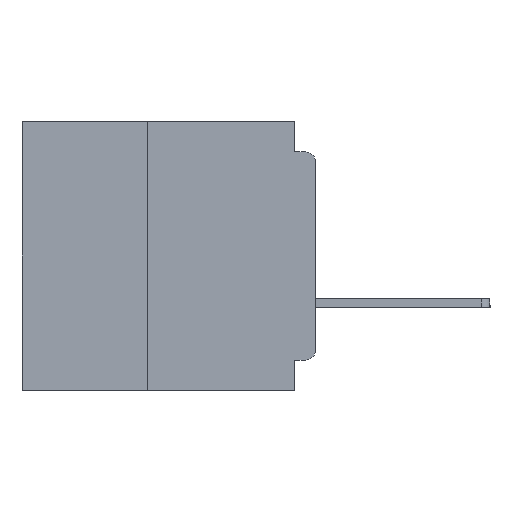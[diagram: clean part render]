
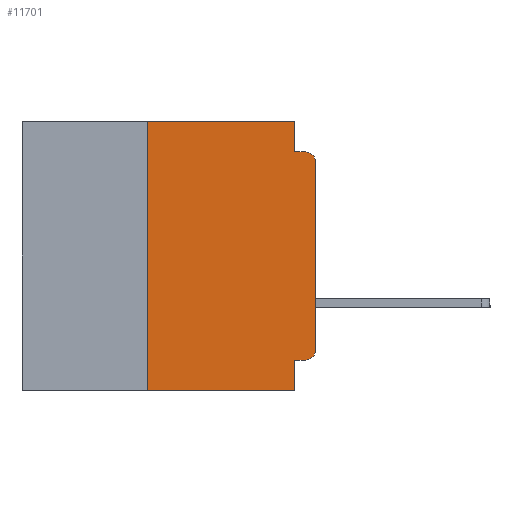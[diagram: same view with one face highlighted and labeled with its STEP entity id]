
A CAD part, left-side view. The second image highlights one B-rep face of the part: STEP entity #11701.
In plain terms, the highlighted planar face has unit normal (-1, 0, 0).
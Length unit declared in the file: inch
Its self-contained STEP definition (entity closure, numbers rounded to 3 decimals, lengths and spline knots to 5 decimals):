
#383 = LINE ( 'NONE', #27352, #30694 ) ;
#846 = EDGE_CURVE ( 'NONE', #26064, #29620, #38356, .T. ) ;
#853 = VERTEX_POINT ( 'NONE', #6180 ) ;
#1189 = EDGE_CURVE ( 'NONE', #33844, #853, #11566, .T. ) ;
#1885 = AXIS2_PLACEMENT_3D ( 'NONE', #35646, #38676, #20667 ) ;
#1981 = EDGE_LOOP ( 'NONE', ( #7978, #34792, #9115, #14322, #16230, #26816, #25661, #27764, #3460, #17053 ) ) ;
#2153 = CARTESIAN_POINT ( 'NONE',  ( 0., 0.015, -0.045 ) ) ;
#2478 = CARTESIAN_POINT ( 'NONE',  ( 0., 0.25, 0. ) ) ;
#3460 = ORIENTED_EDGE ( 'NONE', *, *, #6900, .F. ) ;
#3592 = EDGE_CURVE ( 'NONE', #24916, #29620, #383, .T. ) ;
#4043 = CARTESIAN_POINT ( 'NONE',  ( 0., 0.031, -0.045 ) ) ;
#4719 = VERTEX_POINT ( 'NONE', #2478 ) ;
#5786 = LINE ( 'NONE', #25046, #28989 ) ;
#6180 = CARTESIAN_POINT ( 'NONE',  ( 0., 0., -0.34 ) ) ;
#6378 = CARTESIAN_POINT ( 'NONE',  ( 0., 0.031, -0.4 ) ) ;
#6861 = DIRECTION ( 'NONE',  ( 0., 0., 1. ) ) ;
#6900 = EDGE_CURVE ( 'NONE', #33844, #26064, #34678, .T. ) ;
#7867 = EDGE_CURVE ( 'NONE', #24916, #4719, #5786, .T. ) ;
#7978 = ORIENTED_EDGE ( 'NONE', *, *, #33543, .T. ) ;
#8931 = LINE ( 'NONE', #22292, #24010 ) ;
#9115 = ORIENTED_EDGE ( 'NONE', *, *, #12652, .F. ) ;
#10757 = VERTEX_POINT ( 'NONE', #4043 ) ;
#10973 = CARTESIAN_POINT ( 'NONE',  ( 0., 0.015, -0.34 ) ) ;
#11551 = LINE ( 'NONE', #36520, #18653 ) ;
#11566 = CIRCLE ( 'NONE', #29061, 0.015 ) ;
#11701 = ADVANCED_FACE ( 'NONE', ( #13783 ), #14648, .F. ) ;
#11728 = CARTESIAN_POINT ( 'NONE',  ( 0., 0., -0.355 ) ) ;
#12652 = EDGE_CURVE ( 'NONE', #10757, #16596, #8931, .T. ) ;
#13434 = EDGE_CURVE ( 'NONE', #25987, #16596, #27763, .T. ) ;
#13783 = FACE_OUTER_BOUND ( 'NONE', #1981, .T. ) ;
#14022 = CARTESIAN_POINT ( 'NONE',  ( 0., 0.015, -0.355 ) ) ;
#14029 = DIRECTION ( 'NONE',  ( 0., 0., -1. ) ) ;
#14322 = ORIENTED_EDGE ( 'NONE', *, *, #26779, .F. ) ;
#14519 = CARTESIAN_POINT ( 'NONE',  ( 0., 0., -0.06 ) ) ;
#14648 = PLANE ( 'NONE',  #1885 ) ;
#14652 = DIRECTION ( 'NONE',  ( -1., 0., 0. ) ) ;
#15389 = CARTESIAN_POINT ( 'NONE',  ( 0., 0.031, -0.4 ) ) ;
#16054 = DIRECTION ( 'NONE',  ( 0., 0., 1. ) ) ;
#16230 = ORIENTED_EDGE ( 'NONE', *, *, #27182, .F. ) ;
#16596 = VERTEX_POINT ( 'NONE', #2153 ) ;
#17053 = ORIENTED_EDGE ( 'NONE', *, *, #1189, .T. ) ;
#17940 = CARTESIAN_POINT ( 'NONE',  ( 0., 0.031, -0.355 ) ) ;
#18653 = VECTOR ( 'NONE', #18659, 39.37008 ) ;
#18659 = DIRECTION ( 'NONE',  ( 0., 0., -1. ) ) ;
#18713 = VECTOR ( 'NONE', #20681, 39.37008 ) ;
#20667 = DIRECTION ( 'NONE',  ( 0., 0., -1. ) ) ;
#20681 = DIRECTION ( 'NONE',  ( 0., 1., 0. ) ) ;
#22231 = VECTOR ( 'NONE', #6861, 39.37008 ) ;
#22292 = CARTESIAN_POINT ( 'NONE',  ( 0., 0., -0.045 ) ) ;
#24010 = VECTOR ( 'NONE', #31262, 39.37008 ) ;
#24073 = VECTOR ( 'NONE', #38456, 39.37008 ) ;
#24916 = VERTEX_POINT ( 'NONE', #38907 ) ;
#25010 = LINE ( 'NONE', #35426, #24073 ) ;
#25046 = CARTESIAN_POINT ( 'NONE',  ( 0., 0.25, -0.4 ) ) ;
#25661 = ORIENTED_EDGE ( 'NONE', *, *, #3592, .T. ) ;
#25987 = VERTEX_POINT ( 'NONE', #14519 ) ;
#26064 = VERTEX_POINT ( 'NONE', #17940 ) ;
#26779 = EDGE_CURVE ( 'NONE', #32702, #10757, #11551, .T. ) ;
#26816 = ORIENTED_EDGE ( 'NONE', *, *, #7867, .F. ) ;
#27182 = EDGE_CURVE ( 'NONE', #4719, #32702, #25010, .T. ) ;
#27352 = CARTESIAN_POINT ( 'NONE',  ( 0., 0.437, -0.4 ) ) ;
#27763 = CIRCLE ( 'NONE', #36635, 0.015 ) ;
#27764 = ORIENTED_EDGE ( 'NONE', *, *, #846, .F. ) ;
#28989 = VECTOR ( 'NONE', #16054, 39.37008 ) ;
#29061 = AXIS2_PLACEMENT_3D ( 'NONE', #10973, #32055, #14029 ) ;
#29620 = VERTEX_POINT ( 'NONE', #6378 ) ;
#30694 = VECTOR ( 'NONE', #36388, 39.37008 ) ;
#31011 = CARTESIAN_POINT ( 'NONE',  ( 0., 0., 0. ) ) ;
#31262 = DIRECTION ( 'NONE',  ( 0., -1., 0. ) ) ;
#32055 = DIRECTION ( 'NONE',  ( -1., 0., 0. ) ) ;
#32267 = VECTOR ( 'NONE', #36389, 39.37008 ) ;
#32641 = CARTESIAN_POINT ( 'NONE',  ( 0., 0.015, -0.06 ) ) ;
#32702 = VERTEX_POINT ( 'NONE', #38420 ) ;
#33543 = EDGE_CURVE ( 'NONE', #853, #25987, #39174, .T. ) ;
#33844 = VERTEX_POINT ( 'NONE', #14022 ) ;
#34678 = LINE ( 'NONE', #11728, #18713 ) ;
#34792 = ORIENTED_EDGE ( 'NONE', *, *, #13434, .T. ) ;
#35426 = CARTESIAN_POINT ( 'NONE',  ( 0., 0.437, 0. ) ) ;
#35646 = CARTESIAN_POINT ( 'NONE',  ( 0., 0.437, 0. ) ) ;
#35652 = DIRECTION ( 'NONE',  ( 0., 0., -1. ) ) ;
#36388 = DIRECTION ( 'NONE',  ( 0., -1., 0. ) ) ;
#36389 = DIRECTION ( 'NONE',  ( 0., 0., -1. ) ) ;
#36520 = CARTESIAN_POINT ( 'NONE',  ( 0., 0.031, 0. ) ) ;
#36635 = AXIS2_PLACEMENT_3D ( 'NONE', #32641, #14652, #35652 ) ;
#38356 = LINE ( 'NONE', #15389, #32267 ) ;
#38420 = CARTESIAN_POINT ( 'NONE',  ( 0., 0.031, 0. ) ) ;
#38456 = DIRECTION ( 'NONE',  ( 0., -1., 0. ) ) ;
#38676 = DIRECTION ( 'NONE',  ( 1., 0., 0. ) ) ;
#38907 = CARTESIAN_POINT ( 'NONE',  ( 0., 0.25, -0.4 ) ) ;
#39174 = LINE ( 'NONE', #31011, #22231 ) ;
